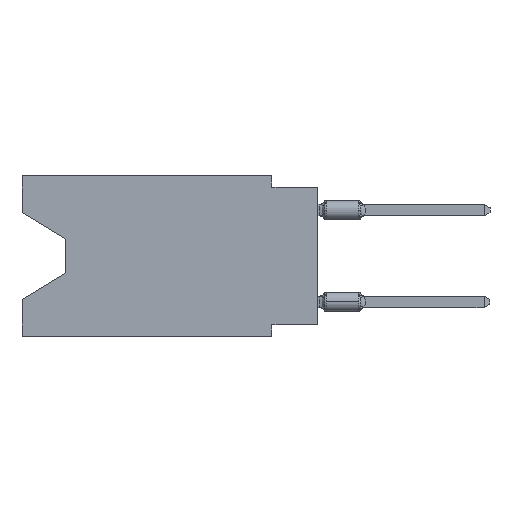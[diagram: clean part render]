
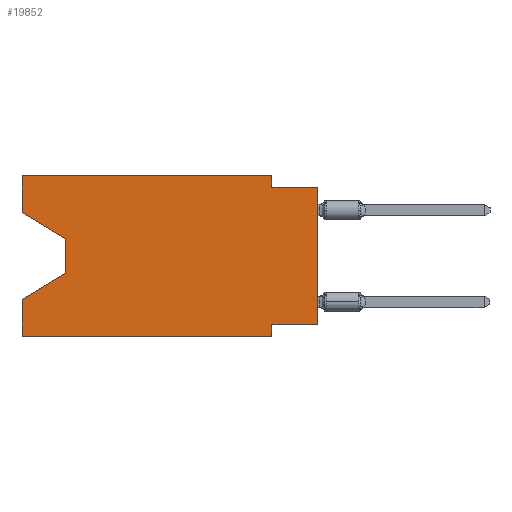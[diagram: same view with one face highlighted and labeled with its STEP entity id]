
A CAD part, left-side view. The second image highlights one B-rep face of the part: STEP entity #19852.
In plain terms, the highlighted planar face has unit normal (-1, 0, 0).
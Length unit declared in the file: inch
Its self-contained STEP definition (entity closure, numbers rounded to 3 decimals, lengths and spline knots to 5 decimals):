
#44 = CARTESIAN_POINT ( 'NONE',  ( 0., 0., 0. ) ) ;
#103 = ORIENTED_EDGE ( 'NONE', *, *, #7525, .F. ) ;
#131 = CARTESIAN_POINT ( 'NONE',  ( 0., 0.645, 0. ) ) ;
#146 = LINE ( 'NONE', #7825, #19750 ) ;
#408 = ORIENTED_EDGE ( 'NONE', *, *, #7885, .F. ) ;
#515 = CARTESIAN_POINT ( 'NONE',  ( 0., 0.1, -0.025 ) ) ;
#568 = CARTESIAN_POINT ( 'NONE',  ( 0., 0.645, 0. ) ) ;
#738 = VERTEX_POINT ( 'NONE', #19685 ) ;
#826 = VECTOR ( 'NONE', #2741, 39.37008 ) ;
#1304 = CARTESIAN_POINT ( 'NONE',  ( 0., 0.1, 0. ) ) ;
#1695 = CARTESIAN_POINT ( 'NONE',  ( 0., 0.645, -0.35 ) ) ;
#1943 = VECTOR ( 'NONE', #18977, 39.37008 ) ;
#2540 = CARTESIAN_POINT ( 'NONE',  ( 0., 0.1, -0.35 ) ) ;
#2686 = VERTEX_POINT ( 'NONE', #15615 ) ;
#2741 = DIRECTION ( 'NONE',  ( 0., 0., -1. ) ) ;
#3064 = LINE ( 'NONE', #44, #13283 ) ;
#3083 = CARTESIAN_POINT ( 'NONE',  ( 0., 0.645, -0.08025 ) ) ;
#3155 = DIRECTION ( 'NONE',  ( 0., 0., 1. ) ) ;
#3335 = VERTEX_POINT ( 'NONE', #3083 ) ;
#3656 = CARTESIAN_POINT ( 'NONE',  ( 0., 0.1, 0. ) ) ;
#4258 = LINE ( 'NONE', #2540, #826 ) ;
#4285 = CARTESIAN_POINT ( 'NONE',  ( 0., 0.55, -0.212 ) ) ;
#5176 = EDGE_CURVE ( 'NONE', #11821, #12011, #8614, .T. ) ;
#5438 = VECTOR ( 'NONE', #5837, 39.37008 ) ;
#5831 = ORIENTED_EDGE ( 'NONE', *, *, #15224, .T. ) ;
#5837 = DIRECTION ( 'NONE',  ( 0., 1., 0. ) ) ;
#6007 = DIRECTION ( 'NONE',  ( 0., 0.855, -0.519 ) ) ;
#6078 = VECTOR ( 'NONE', #15746, 39.37008 ) ;
#6232 = EDGE_CURVE ( 'NONE', #738, #17085, #18473, .T. ) ;
#6613 = DIRECTION ( 'NONE',  ( 0., -1., 0. ) ) ;
#6746 = AXIS2_PLACEMENT_3D ( 'NONE', #131, #8006, #11150 ) ;
#7092 = VECTOR ( 'NONE', #14157, 39.37008 ) ;
#7255 = CARTESIAN_POINT ( 'NONE',  ( 0., 0., -0.325 ) ) ;
#7525 = EDGE_CURVE ( 'NONE', #16347, #17721, #8554, .T. ) ;
#7557 = LINE ( 'NONE', #1695, #6078 ) ;
#7678 = VERTEX_POINT ( 'NONE', #13961 ) ;
#7825 = CARTESIAN_POINT ( 'NONE',  ( 0., 0.645, 0. ) ) ;
#7885 = EDGE_CURVE ( 'NONE', #18599, #16347, #14464, .T. ) ;
#8006 = DIRECTION ( 'NONE',  ( 1., 0., 0. ) ) ;
#8162 = VECTOR ( 'NONE', #14329, 39.37008 ) ;
#8192 = CARTESIAN_POINT ( 'NONE',  ( 0., 0.645, 0. ) ) ;
#8358 = ORIENTED_EDGE ( 'NONE', *, *, #10006, .F. ) ;
#8554 = LINE ( 'NONE', #19273, #1943 ) ;
#8614 = LINE ( 'NONE', #17453, #12573 ) ;
#8759 = CARTESIAN_POINT ( 'NONE',  ( 0., 0.55, -0.212 ) ) ;
#9405 = VERTEX_POINT ( 'NONE', #11869 ) ;
#9515 = EDGE_CURVE ( 'NONE', #2686, #18599, #146, .T. ) ;
#9598 = EDGE_CURVE ( 'NONE', #738, #17721, #3064, .T. ) ;
#9767 = DIRECTION ( 'NONE',  ( 0., 0., -1. ) ) ;
#9790 = VECTOR ( 'NONE', #18650, 39.37008 ) ;
#10006 = EDGE_CURVE ( 'NONE', #3335, #2686, #12713, .T. ) ;
#10137 = LINE ( 'NONE', #19722, #11462 ) ;
#10422 = EDGE_CURVE ( 'NONE', #9405, #17333, #12480, .T. ) ;
#10605 = ORIENTED_EDGE ( 'NONE', *, *, #6232, .F. ) ;
#10842 = PLANE ( 'NONE',  #6746 ) ;
#11150 = DIRECTION ( 'NONE',  ( 0., 0., -1. ) ) ;
#11462 = VECTOR ( 'NONE', #13253, 39.37008 ) ;
#11821 = VERTEX_POINT ( 'NONE', #18642 ) ;
#11869 = CARTESIAN_POINT ( 'NONE',  ( 0., 0.645, -0.35 ) ) ;
#11898 = ORIENTED_EDGE ( 'NONE', *, *, #16066, .T. ) ;
#12011 = VERTEX_POINT ( 'NONE', #4285 ) ;
#12480 = LINE ( 'NONE', #568, #9790 ) ;
#12573 = VECTOR ( 'NONE', #9767, 39.37008 ) ;
#12713 = LINE ( 'NONE', #8192, #8162 ) ;
#13253 = DIRECTION ( 'NONE',  ( 0., -0.855, -0.519 ) ) ;
#13283 = VECTOR ( 'NONE', #3155, 39.37008 ) ;
#13343 = EDGE_LOOP ( 'NONE', ( #11898, #14162, #5831, #19382, #17435, #17673, #10605, #17216, #103, #408, #15648, #8358 ) ) ;
#13961 = CARTESIAN_POINT ( 'NONE',  ( 0., 0.1, -0.35 ) ) ;
#14157 = DIRECTION ( 'NONE',  ( 0., 0., -1. ) ) ;
#14162 = ORIENTED_EDGE ( 'NONE', *, *, #5176, .T. ) ;
#14329 = DIRECTION ( 'NONE',  ( 0., 0., 1. ) ) ;
#14464 = LINE ( 'NONE', #3656, #7092 ) ;
#15224 = EDGE_CURVE ( 'NONE', #12011, #17333, #18146, .T. ) ;
#15523 = CARTESIAN_POINT ( 'NONE',  ( 0., 0.645, -0.26975 ) ) ;
#15615 = CARTESIAN_POINT ( 'NONE',  ( 0., 0.645, 0. ) ) ;
#15648 = ORIENTED_EDGE ( 'NONE', *, *, #9515, .F. ) ;
#15746 = DIRECTION ( 'NONE',  ( 0., -1., 0. ) ) ;
#16050 = CARTESIAN_POINT ( 'NONE',  ( 0., 0.1, -0.325 ) ) ;
#16066 = EDGE_CURVE ( 'NONE', #3335, #11821, #10137, .T. ) ;
#16347 = VERTEX_POINT ( 'NONE', #515 ) ;
#17085 = VERTEX_POINT ( 'NONE', #16050 ) ;
#17112 = FACE_OUTER_BOUND ( 'NONE', #13343, .T. ) ;
#17216 = ORIENTED_EDGE ( 'NONE', *, *, #9598, .T. ) ;
#17333 = VERTEX_POINT ( 'NONE', #15523 ) ;
#17435 = ORIENTED_EDGE ( 'NONE', *, *, #19415, .T. ) ;
#17453 = CARTESIAN_POINT ( 'NONE',  ( 0., 0.55, -0.138 ) ) ;
#17673 = ORIENTED_EDGE ( 'NONE', *, *, #18015, .F. ) ;
#17721 = VERTEX_POINT ( 'NONE', #18728 ) ;
#17768 = VECTOR ( 'NONE', #6007, 39.37008 ) ;
#18015 = EDGE_CURVE ( 'NONE', #17085, #7678, #4258, .T. ) ;
#18146 = LINE ( 'NONE', #8759, #17768 ) ;
#18473 = LINE ( 'NONE', #7255, #5438 ) ;
#18599 = VERTEX_POINT ( 'NONE', #1304 ) ;
#18642 = CARTESIAN_POINT ( 'NONE',  ( 0., 0.55, -0.138 ) ) ;
#18650 = DIRECTION ( 'NONE',  ( 0., 0., 1. ) ) ;
#18728 = CARTESIAN_POINT ( 'NONE',  ( 0., 0., -0.025 ) ) ;
#18977 = DIRECTION ( 'NONE',  ( 0., -1., 0. ) ) ;
#19273 = CARTESIAN_POINT ( 'NONE',  ( 0., 0., -0.025 ) ) ;
#19382 = ORIENTED_EDGE ( 'NONE', *, *, #10422, .F. ) ;
#19415 = EDGE_CURVE ( 'NONE', #9405, #7678, #7557, .T. ) ;
#19685 = CARTESIAN_POINT ( 'NONE',  ( 0., 0., -0.325 ) ) ;
#19722 = CARTESIAN_POINT ( 'NONE',  ( 0., 0.645, -0.08025 ) ) ;
#19750 = VECTOR ( 'NONE', #6613, 39.37008 ) ;
#19852 = ADVANCED_FACE ( 'NONE', ( #17112 ), #10842, .F. ) ;
